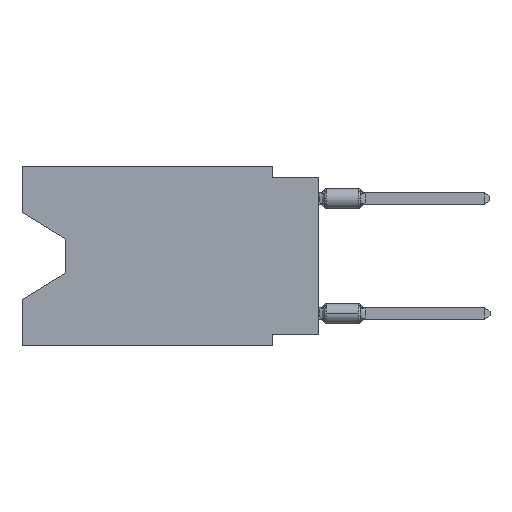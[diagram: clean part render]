
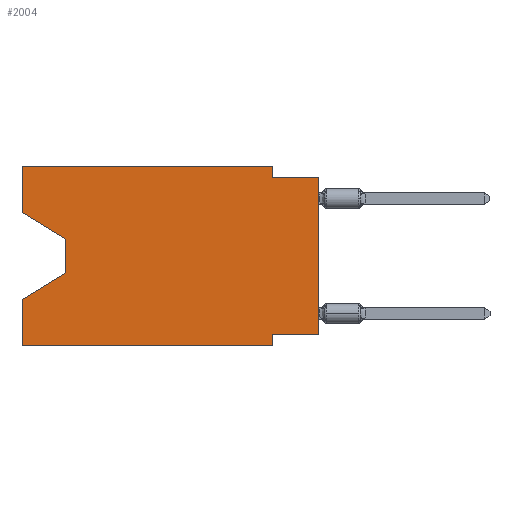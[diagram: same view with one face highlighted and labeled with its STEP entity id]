
A CAD part, left-side view. The second image highlights one B-rep face of the part: STEP entity #2004.
In plain terms, the highlighted planar face has unit normal (-1, 0, 0).
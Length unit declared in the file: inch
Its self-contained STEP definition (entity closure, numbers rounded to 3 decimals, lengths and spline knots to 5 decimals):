
#208 = CARTESIAN_POINT ( 'NONE',  ( 0., 0.645, 0. ) ) ;
#302 = EDGE_CURVE ( 'NONE', #320, #18959, #12690, .T. ) ;
#320 = VERTEX_POINT ( 'NONE', #14849 ) ;
#661 = VERTEX_POINT ( 'NONE', #12669 ) ;
#875 = CARTESIAN_POINT ( 'NONE',  ( 0., 0.645, -0.39 ) ) ;
#910 = CARTESIAN_POINT ( 'NONE',  ( 0., 0., -0.365 ) ) ;
#1288 = VECTOR ( 'NONE', #7934, 39.37008 ) ;
#1455 = DIRECTION ( 'NONE',  ( 0., -1., 0. ) ) ;
#1543 = AXIS2_PLACEMENT_3D ( 'NONE', #208, #10125, #15350 ) ;
#1603 = ORIENTED_EDGE ( 'NONE', *, *, #18407, .F. ) ;
#1699 = EDGE_CURVE ( 'NONE', #8036, #15180, #16887, .T. ) ;
#1811 = PLANE ( 'NONE',  #1543 ) ;
#2004 = ADVANCED_FACE ( 'NONE', ( #12093 ), #1811, .F. ) ;
#2013 = LINE ( 'NONE', #20008, #12063 ) ;
#2465 = ORIENTED_EDGE ( 'NONE', *, *, #20661, .T. ) ;
#2466 = ORIENTED_EDGE ( 'NONE', *, *, #17234, .F. ) ;
#2714 = VECTOR ( 'NONE', #17775, 39.37008 ) ;
#2797 = CARTESIAN_POINT ( 'NONE',  ( 0., 0.645, 0. ) ) ;
#2799 = VECTOR ( 'NONE', #4400, 39.37008 ) ;
#2910 = ORIENTED_EDGE ( 'NONE', *, *, #4261, .T. ) ;
#3919 = VECTOR ( 'NONE', #1455, 39.37008 ) ;
#4013 = DIRECTION ( 'NONE',  ( 0., 0., 1. ) ) ;
#4046 = LINE ( 'NONE', #9058, #7493 ) ;
#4217 = LINE ( 'NONE', #7483, #17218 ) ;
#4261 = EDGE_CURVE ( 'NONE', #7079, #661, #17267, .T. ) ;
#4400 = DIRECTION ( 'NONE',  ( 0., 0., 1. ) ) ;
#5118 = VERTEX_POINT ( 'NONE', #20362 ) ;
#5297 = CARTESIAN_POINT ( 'NONE',  ( 0., 0.1, -0.365 ) ) ;
#5386 = VECTOR ( 'NONE', #12698, 39.37008 ) ;
#5498 = DIRECTION ( 'NONE',  ( 0., 0., -1. ) ) ;
#5577 = DIRECTION ( 'NONE',  ( 0., 0., -1. ) ) ;
#5922 = CARTESIAN_POINT ( 'NONE',  ( 0., 0.1, -0.39 ) ) ;
#6025 = CARTESIAN_POINT ( 'NONE',  ( 0., 0.55, -0.158 ) ) ;
#6066 = EDGE_CURVE ( 'NONE', #15042, #6915, #9424, .T. ) ;
#6483 = EDGE_CURVE ( 'NONE', #13719, #320, #19184, .T. ) ;
#6915 = VERTEX_POINT ( 'NONE', #5922 ) ;
#7079 = VERTEX_POINT ( 'NONE', #17278 ) ;
#7109 = ORIENTED_EDGE ( 'NONE', *, *, #14410, .F. ) ;
#7412 = ORIENTED_EDGE ( 'NONE', *, *, #6483, .F. ) ;
#7483 = CARTESIAN_POINT ( 'NONE',  ( 0., 0.55, -0.232 ) ) ;
#7493 = VECTOR ( 'NONE', #15685, 39.37008 ) ;
#7934 = DIRECTION ( 'NONE',  ( 0., 0., 1. ) ) ;
#8036 = VERTEX_POINT ( 'NONE', #6025 ) ;
#8601 = DIRECTION ( 'NONE',  ( 0., -0.855, -0.519 ) ) ;
#8937 = EDGE_CURVE ( 'NONE', #7079, #13460, #10968, .T. ) ;
#9058 = CARTESIAN_POINT ( 'NONE',  ( 0., 0.1, 0. ) ) ;
#9424 = LINE ( 'NONE', #21237, #5386 ) ;
#9425 = DIRECTION ( 'NONE',  ( 0., 1., 0. ) ) ;
#10065 = VECTOR ( 'NONE', #5498, 39.37008 ) ;
#10125 = DIRECTION ( 'NONE',  ( 1., 0., 0. ) ) ;
#10347 = CARTESIAN_POINT ( 'NONE',  ( 0., 0.645, -0.10025 ) ) ;
#10968 = LINE ( 'NONE', #910, #13181 ) ;
#10987 = CARTESIAN_POINT ( 'NONE',  ( 0., 0., -0.025 ) ) ;
#11085 = LINE ( 'NONE', #10987, #3919 ) ;
#11507 = ORIENTED_EDGE ( 'NONE', *, *, #18706, .T. ) ;
#11699 = CARTESIAN_POINT ( 'NONE',  ( 0., 0.1, 0. ) ) ;
#12063 = VECTOR ( 'NONE', #8601, 39.37008 ) ;
#12093 = FACE_OUTER_BOUND ( 'NONE', #16965, .T. ) ;
#12456 = VERTEX_POINT ( 'NONE', #13603 ) ;
#12669 = CARTESIAN_POINT ( 'NONE',  ( 0., 0., -0.025 ) ) ;
#12690 = LINE ( 'NONE', #14412, #2714 ) ;
#12698 = DIRECTION ( 'NONE',  ( 0., -1., 0. ) ) ;
#13181 = VECTOR ( 'NONE', #9425, 39.37008 ) ;
#13337 = ORIENTED_EDGE ( 'NONE', *, *, #302, .F. ) ;
#13460 = VERTEX_POINT ( 'NONE', #5297 ) ;
#13603 = CARTESIAN_POINT ( 'NONE',  ( 0., 0.645, -0.28975 ) ) ;
#13719 = VERTEX_POINT ( 'NONE', #10347 ) ;
#13812 = CARTESIAN_POINT ( 'NONE',  ( 0., 0.1, -0.39 ) ) ;
#13924 = LINE ( 'NONE', #13812, #19657 ) ;
#14410 = EDGE_CURVE ( 'NONE', #5118, #661, #11085, .T. ) ;
#14412 = CARTESIAN_POINT ( 'NONE',  ( 0., 0.645, 0. ) ) ;
#14849 = CARTESIAN_POINT ( 'NONE',  ( 0., 0.645, 0. ) ) ;
#15042 = VERTEX_POINT ( 'NONE', #875 ) ;
#15054 = ORIENTED_EDGE ( 'NONE', *, *, #8937, .F. ) ;
#15180 = VERTEX_POINT ( 'NONE', #19176 ) ;
#15350 = DIRECTION ( 'NONE',  ( 0., 0., -1. ) ) ;
#15653 = ORIENTED_EDGE ( 'NONE', *, *, #6066, .T. ) ;
#15685 = DIRECTION ( 'NONE',  ( 0., 0., -1. ) ) ;
#16194 = ORIENTED_EDGE ( 'NONE', *, *, #1699, .T. ) ;
#16887 = LINE ( 'NONE', #20146, #10065 ) ;
#16965 = EDGE_LOOP ( 'NONE', ( #2465, #16194, #11507, #2466, #15653, #20632, #15054, #2910, #7109, #1603, #13337, #7412 ) ) ;
#17218 = VECTOR ( 'NONE', #19214, 39.37008 ) ;
#17234 = EDGE_CURVE ( 'NONE', #15042, #12456, #19857, .T. ) ;
#17267 = LINE ( 'NONE', #18918, #19045 ) ;
#17278 = CARTESIAN_POINT ( 'NONE',  ( 0., 0., -0.365 ) ) ;
#17775 = DIRECTION ( 'NONE',  ( 0., -1., 0. ) ) ;
#18229 = CARTESIAN_POINT ( 'NONE',  ( 0., 0.645, 0. ) ) ;
#18407 = EDGE_CURVE ( 'NONE', #18959, #5118, #4046, .T. ) ;
#18706 = EDGE_CURVE ( 'NONE', #15180, #12456, #4217, .T. ) ;
#18918 = CARTESIAN_POINT ( 'NONE',  ( 0., 0., 0. ) ) ;
#18959 = VERTEX_POINT ( 'NONE', #11699 ) ;
#19045 = VECTOR ( 'NONE', #4013, 39.37008 ) ;
#19176 = CARTESIAN_POINT ( 'NONE',  ( 0., 0.55, -0.232 ) ) ;
#19184 = LINE ( 'NONE', #2797, #2799 ) ;
#19214 = DIRECTION ( 'NONE',  ( 0., 0.855, -0.519 ) ) ;
#19605 = EDGE_CURVE ( 'NONE', #13460, #6915, #13924, .T. ) ;
#19657 = VECTOR ( 'NONE', #5577, 39.37008 ) ;
#19857 = LINE ( 'NONE', #18229, #1288 ) ;
#20008 = CARTESIAN_POINT ( 'NONE',  ( 0., 0.645, -0.10025 ) ) ;
#20146 = CARTESIAN_POINT ( 'NONE',  ( 0., 0.55, -0.158 ) ) ;
#20362 = CARTESIAN_POINT ( 'NONE',  ( 0., 0.1, -0.025 ) ) ;
#20632 = ORIENTED_EDGE ( 'NONE', *, *, #19605, .F. ) ;
#20661 = EDGE_CURVE ( 'NONE', #13719, #8036, #2013, .T. ) ;
#21237 = CARTESIAN_POINT ( 'NONE',  ( 0., 0.645, -0.39 ) ) ;
